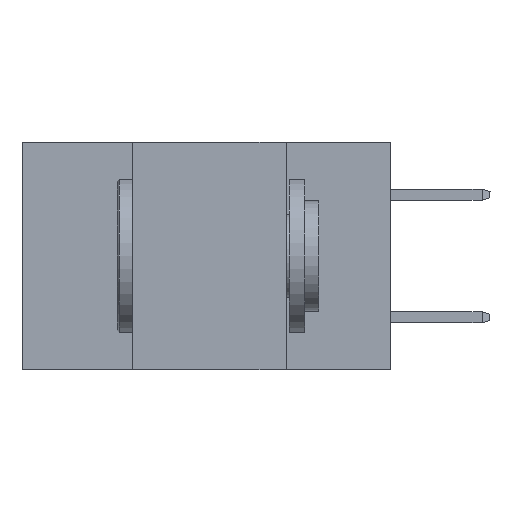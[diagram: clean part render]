
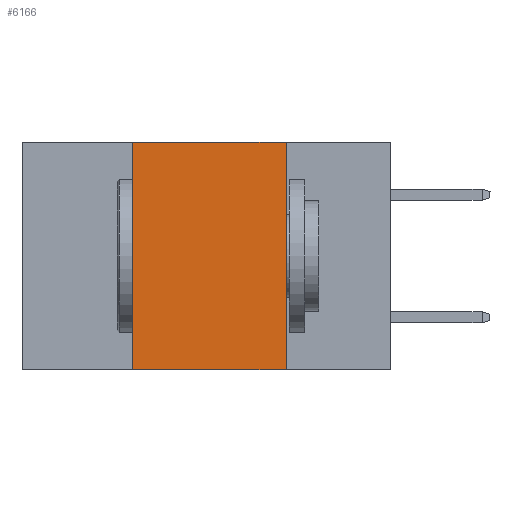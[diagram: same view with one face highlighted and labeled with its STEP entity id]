
A CAD part, left-side view. The second image highlights one B-rep face of the part: STEP entity #6166.
In plain terms, the highlighted planar face has unit normal (-1, 0, 0).
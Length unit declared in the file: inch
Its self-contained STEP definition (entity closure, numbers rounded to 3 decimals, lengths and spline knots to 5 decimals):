
#257 = DIRECTION ( 'NONE',  ( 0., -1., 0. ) ) ;
#418 = LINE ( 'NONE', #6789, #3965 ) ;
#913 = EDGE_CURVE ( 'NONE', #5859, #5344, #4498, .T. ) ;
#1095 = CARTESIAN_POINT ( 'NONE',  ( 0., 0.6, 0. ) ) ;
#1113 = VERTEX_POINT ( 'NONE', #10052 ) ;
#1268 = ORIENTED_EDGE ( 'NONE', *, *, #5588, .F. ) ;
#1387 = ORIENTED_EDGE ( 'NONE', *, *, #4049, .T. ) ;
#1473 = LINE ( 'NONE', #7453, #10826 ) ;
#1947 = FACE_OUTER_BOUND ( 'NONE', #6058, .T. ) ;
#2097 = VECTOR ( 'NONE', #11678, 39.37008 ) ;
#3098 = ORIENTED_EDGE ( 'NONE', *, *, #913, .F. ) ;
#3327 = CARTESIAN_POINT ( 'NONE',  ( 0., 0.42, -0.37 ) ) ;
#3761 = AXIS2_PLACEMENT_3D ( 'NONE', #9085, #10909, #5691 ) ;
#3965 = VECTOR ( 'NONE', #8497, 39.37008 ) ;
#4049 = EDGE_CURVE ( 'NONE', #5859, #7113, #1473, .T. ) ;
#4498 = LINE ( 'NONE', #8983, #2097 ) ;
#4618 = LINE ( 'NONE', #1095, #11016 ) ;
#5344 = VERTEX_POINT ( 'NONE', #9927 ) ;
#5588 = EDGE_CURVE ( 'NONE', #5344, #1113, #4618, .T. ) ;
#5691 = DIRECTION ( 'NONE',  ( 0., 0., -1. ) ) ;
#5859 = VERTEX_POINT ( 'NONE', #3327 ) ;
#6058 = EDGE_LOOP ( 'NONE', ( #8579, #1268, #3098, #1387 ) ) ;
#6163 = CARTESIAN_POINT ( 'NONE',  ( 0., 0.17, -0.37 ) ) ;
#6166 = ADVANCED_FACE ( 'NONE', ( #1947 ), #6713, .F. ) ;
#6713 = PLANE ( 'NONE',  #3761 ) ;
#6789 = CARTESIAN_POINT ( 'NONE',  ( 0., 0.17, 0. ) ) ;
#7113 = VERTEX_POINT ( 'NONE', #6163 ) ;
#7453 = CARTESIAN_POINT ( 'NONE',  ( 0., 0.6, -0.37 ) ) ;
#7512 = DIRECTION ( 'NONE',  ( 0., -1., 0. ) ) ;
#8497 = DIRECTION ( 'NONE',  ( 0., 0., -1. ) ) ;
#8579 = ORIENTED_EDGE ( 'NONE', *, *, #10478, .F. ) ;
#8983 = CARTESIAN_POINT ( 'NONE',  ( 0., 0.42, 0. ) ) ;
#9085 = CARTESIAN_POINT ( 'NONE',  ( 0., 0.6, 0. ) ) ;
#9927 = CARTESIAN_POINT ( 'NONE',  ( 0., 0.42, 0. ) ) ;
#10052 = CARTESIAN_POINT ( 'NONE',  ( 0., 0.17, 0. ) ) ;
#10478 = EDGE_CURVE ( 'NONE', #1113, #7113, #418, .T. ) ;
#10826 = VECTOR ( 'NONE', #257, 39.37008 ) ;
#10909 = DIRECTION ( 'NONE',  ( 1., 0., 0. ) ) ;
#11016 = VECTOR ( 'NONE', #7512, 39.37008 ) ;
#11678 = DIRECTION ( 'NONE',  ( 0., 0., 1. ) ) ;
